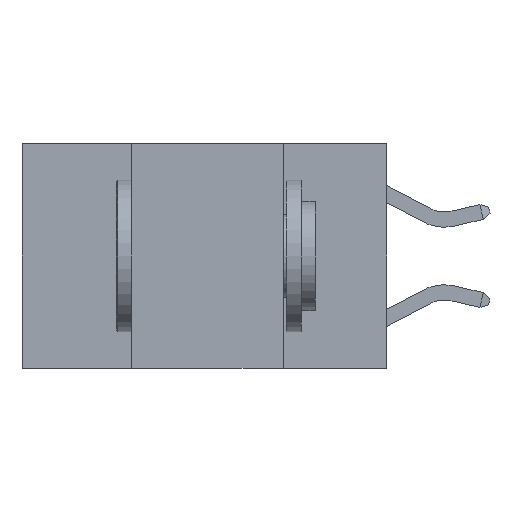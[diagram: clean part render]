
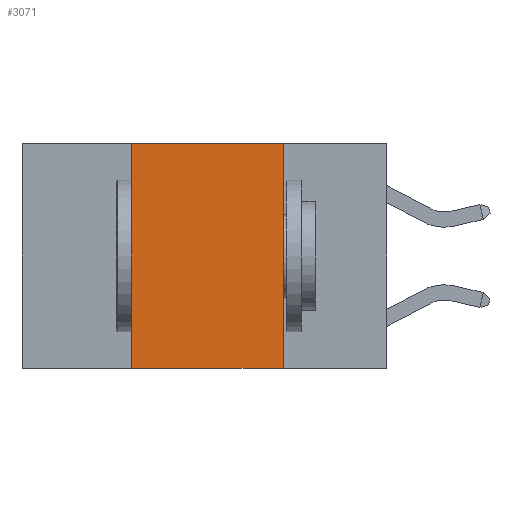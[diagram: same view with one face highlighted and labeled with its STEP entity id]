
A CAD part, left-side view. The second image highlights one B-rep face of the part: STEP entity #3071.
In plain terms, the highlighted planar face has unit normal (-1, 0, 0).
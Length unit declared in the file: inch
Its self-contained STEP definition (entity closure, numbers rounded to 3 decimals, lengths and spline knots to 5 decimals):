
#197 = ORIENTED_EDGE ( 'NONE', *, *, #2948, .T. ) ;
#219 = VECTOR ( 'NONE', #5566, 39.37008 ) ;
#664 = DIRECTION ( 'NONE',  ( 1., 0., 0. ) ) ;
#758 = LINE ( 'NONE', #1959, #2783 ) ;
#1618 = VERTEX_POINT ( 'NONE', #9018 ) ;
#1959 = CARTESIAN_POINT ( 'NONE',  ( 0., 0.6, 0. ) ) ;
#2270 = LINE ( 'NONE', #4689, #219 ) ;
#2406 = FACE_OUTER_BOUND ( 'NONE', #4817, .T. ) ;
#2418 = LINE ( 'NONE', #2709, #8435 ) ;
#2709 = CARTESIAN_POINT ( 'NONE',  ( 0., 0.42, 0. ) ) ;
#2783 = VECTOR ( 'NONE', #2812, 39.37008 ) ;
#2812 = DIRECTION ( 'NONE',  ( 0., -1., 0. ) ) ;
#2813 = EDGE_CURVE ( 'NONE', #7188, #1618, #2418, .T. ) ;
#2822 = DIRECTION ( 'NONE',  ( 0., 0., -1. ) ) ;
#2948 = EDGE_CURVE ( 'NONE', #7188, #3621, #2270, .T. ) ;
#3071 = ADVANCED_FACE ( 'NONE', ( #2406 ), #9951, .F. ) ;
#3165 = CARTESIAN_POINT ( 'NONE',  ( 0., 0.42, -0.37 ) ) ;
#3573 = DIRECTION ( 'NONE',  ( 0., 0., 1. ) ) ;
#3621 = VERTEX_POINT ( 'NONE', #6822 ) ;
#3725 = EDGE_CURVE ( 'NONE', #1618, #9636, #758, .T. ) ;
#4570 = CARTESIAN_POINT ( 'NONE',  ( 0., 0.17, 0. ) ) ;
#4689 = CARTESIAN_POINT ( 'NONE',  ( 0., 0.6, -0.37 ) ) ;
#4817 = EDGE_LOOP ( 'NONE', ( #8837, #9676, #8316, #197 ) ) ;
#5535 = EDGE_CURVE ( 'NONE', #9636, #3621, #8456, .T. ) ;
#5566 = DIRECTION ( 'NONE',  ( 0., -1., 0. ) ) ;
#5859 = CARTESIAN_POINT ( 'NONE',  ( 0., 0.6, 0. ) ) ;
#6411 = VECTOR ( 'NONE', #2822, 39.37008 ) ;
#6598 = DIRECTION ( 'NONE',  ( 0., 0., -1. ) ) ;
#6822 = CARTESIAN_POINT ( 'NONE',  ( 0., 0.17, -0.37 ) ) ;
#7188 = VERTEX_POINT ( 'NONE', #3165 ) ;
#7655 = AXIS2_PLACEMENT_3D ( 'NONE', #5859, #664, #6598 ) ;
#8285 = CARTESIAN_POINT ( 'NONE',  ( 0., 0.17, 0. ) ) ;
#8316 = ORIENTED_EDGE ( 'NONE', *, *, #2813, .F. ) ;
#8435 = VECTOR ( 'NONE', #3573, 39.37008 ) ;
#8456 = LINE ( 'NONE', #4570, #6411 ) ;
#8837 = ORIENTED_EDGE ( 'NONE', *, *, #5535, .F. ) ;
#9018 = CARTESIAN_POINT ( 'NONE',  ( 0., 0.42, 0. ) ) ;
#9636 = VERTEX_POINT ( 'NONE', #8285 ) ;
#9676 = ORIENTED_EDGE ( 'NONE', *, *, #3725, .F. ) ;
#9951 = PLANE ( 'NONE',  #7655 ) ;
